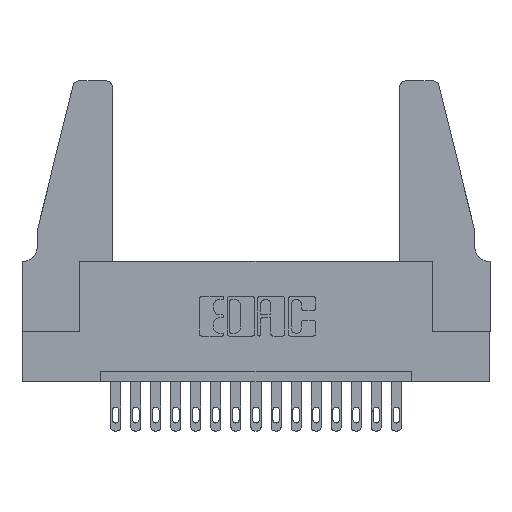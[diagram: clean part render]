
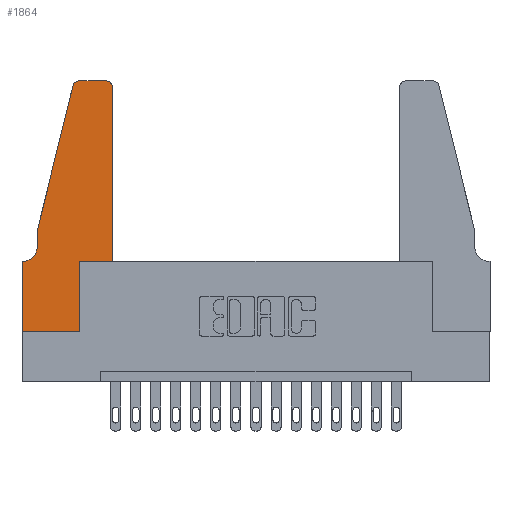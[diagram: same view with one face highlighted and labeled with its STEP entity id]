
A CAD part, top view. The second image highlights one B-rep face of the part: STEP entity #1864.
In plain terms, the highlighted planar face has unit normal (0, 0, 1).
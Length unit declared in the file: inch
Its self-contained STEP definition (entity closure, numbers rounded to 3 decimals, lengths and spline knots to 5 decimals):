
#254 = DIRECTION ( 'NONE',  ( 0., 1., 0. ) ) ;
#261 = VERTEX_POINT ( 'NONE', #9381 ) ;
#372 = VECTOR ( 'NONE', #9721, 39.37008 ) ;
#529 = EDGE_CURVE ( 'NONE', #10047, #14169, #13421, .T. ) ;
#622 = ORIENTED_EDGE ( 'NONE', *, *, #4790, .T. ) ;
#1301 = VERTEX_POINT ( 'NONE', #7020 ) ;
#1384 = CARTESIAN_POINT ( 'NONE',  ( 0.4505, 0.35, 0.37 ) ) ;
#1813 = LINE ( 'NONE', #4146, #16368 ) ;
#1864 = ADVANCED_FACE ( 'NONE', ( #2322 ), #10809, .T. ) ;
#1888 = DIRECTION ( 'NONE',  ( 0., -1., 0. ) ) ;
#2164 = DIRECTION ( 'NONE',  ( 0., 0., 1. ) ) ;
#2322 = FACE_OUTER_BOUND ( 'NONE', #7663, .T. ) ;
#2970 = DIRECTION ( 'NONE',  ( 1., 0., 0. ) ) ;
#3041 = VECTOR ( 'NONE', #2970, 39.37008 ) ;
#3191 = DIRECTION ( 'NONE',  ( 0., -1., 0. ) ) ;
#3827 = VERTEX_POINT ( 'NONE', #16383 ) ;
#4038 = CARTESIAN_POINT ( 'NONE',  ( 0.0755, 0.35, 0.37 ) ) ;
#4050 = VECTOR ( 'NONE', #8361, 39.37008 ) ;
#4146 = CARTESIAN_POINT ( 'NONE',  ( 0.2865, 0.35, 0.37 ) ) ;
#4230 = DIRECTION ( 'NONE',  ( 0., 0., 1. ) ) ;
#4712 = CIRCLE ( 'NONE', #5655, 0.07 ) ;
#4785 = EDGE_CURVE ( 'NONE', #4840, #15629, #5254, .T. ) ;
#4790 = EDGE_CURVE ( 'NONE', #15629, #10047, #1813, .T. ) ;
#4840 = VERTEX_POINT ( 'NONE', #9409 ) ;
#4907 = ORIENTED_EDGE ( 'NONE', *, *, #15145, .T. ) ;
#5006 = CARTESIAN_POINT ( 'NONE',  ( 0.4205, 1.22, 0.37 ) ) ;
#5213 = EDGE_CURVE ( 'NONE', #14169, #13486, #7251, .T. ) ;
#5254 = LINE ( 'NONE', #16036, #3041 ) ;
#5362 = DIRECTION ( 'NONE',  ( -1., 0., 0. ) ) ;
#5575 = ORIENTED_EDGE ( 'NONE', *, *, #11340, .T. ) ;
#5655 = AXIS2_PLACEMENT_3D ( 'NONE', #9706, #11009, #12337 ) ;
#5667 = CIRCLE ( 'NONE', #8144, 0.03 ) ;
#5766 = CARTESIAN_POINT ( 'NONE',  ( 0.25487, 1.22718, 0.37 ) ) ;
#6343 = ORIENTED_EDGE ( 'NONE', *, *, #11801, .T. ) ;
#6541 = EDGE_CURVE ( 'NONE', #15241, #4840, #14198, .T. ) ;
#6826 = ORIENTED_EDGE ( 'NONE', *, *, #14881, .T. ) ;
#7020 = CARTESIAN_POINT ( 'NONE',  ( 0.0055, 0.35, 0.37 ) ) ;
#7075 = CARTESIAN_POINT ( 'NONE',  ( 0.4205, 1.25, 0.37 ) ) ;
#7163 = CIRCLE ( 'NONE', #14122, 0.03 ) ;
#7246 = CARTESIAN_POINT ( 'NONE',  ( 0.2605, 1.25, 0.37 ) ) ;
#7251 = LINE ( 'NONE', #10369, #13852 ) ;
#7286 = CARTESIAN_POINT ( 'NONE',  ( 0.284, 1.22, 0.37 ) ) ;
#7649 = CARTESIAN_POINT ( 'NONE',  ( 0.4505, 1.22, 0.37 ) ) ;
#7663 = EDGE_LOOP ( 'NONE', ( #6343, #15482, #5575, #4907, #11288, #6826, #15366, #9174, #622, #8635, #10661, #15835 ) ) ;
#8144 = AXIS2_PLACEMENT_3D ( 'NONE', #5006, #11484, #16696 ) ;
#8361 = DIRECTION ( 'NONE',  ( -0.239, -0.971, 0. ) ) ;
#8538 = CARTESIAN_POINT ( 'NONE',  ( 0.0755, 0.5, 0.37 ) ) ;
#8635 = ORIENTED_EDGE ( 'NONE', *, *, #529, .T. ) ;
#8824 = LINE ( 'NONE', #8538, #16271 ) ;
#9174 = ORIENTED_EDGE ( 'NONE', *, *, #4785, .T. ) ;
#9213 = CARTESIAN_POINT ( 'NONE',  ( 0., 0.35, 0.37 ) ) ;
#9381 = CARTESIAN_POINT ( 'NONE',  ( 0.284, 1.25, 0.37 ) ) ;
#9409 = CARTESIAN_POINT ( 'NONE',  ( 0., 0., 0.37 ) ) ;
#9539 = CARTESIAN_POINT ( 'NONE',  ( 0.0755, 0.5, 0.37 ) ) ;
#9706 = CARTESIAN_POINT ( 'NONE',  ( 0.0055, 0.42, 0.37 ) ) ;
#9721 = DIRECTION ( 'NONE',  ( -1., 0., 0. ) ) ;
#9727 = CARTESIAN_POINT ( 'NONE',  ( 0.2865, 0., 0.37 ) ) ;
#10047 = VERTEX_POINT ( 'NONE', #16821 ) ;
#10242 = EDGE_CURVE ( 'NONE', #13486, #16090, #5667, .T. ) ;
#10304 = VECTOR ( 'NONE', #13217, 39.37008 ) ;
#10369 = CARTESIAN_POINT ( 'NONE',  ( 0.4505, 0.35, 0.37 ) ) ;
#10422 = DIRECTION ( 'NONE',  ( 0., 1., 0. ) ) ;
#10661 = ORIENTED_EDGE ( 'NONE', *, *, #5213, .T. ) ;
#10676 = VECTOR ( 'NONE', #3191, 39.37008 ) ;
#10809 = PLANE ( 'NONE',  #11166 ) ;
#10815 = LINE ( 'NONE', #9539, #4050 ) ;
#10983 = CARTESIAN_POINT ( 'NONE',  ( 0., 0.35, 0.37 ) ) ;
#11009 = DIRECTION ( 'NONE',  ( 0., 0., -1. ) ) ;
#11166 = AXIS2_PLACEMENT_3D ( 'NONE', #10983, #4230, #12257 ) ;
#11288 = ORIENTED_EDGE ( 'NONE', *, *, #15777, .T. ) ;
#11340 = EDGE_CURVE ( 'NONE', #13668, #3827, #10815, .T. ) ;
#11484 = DIRECTION ( 'NONE',  ( 0., 0., 1. ) ) ;
#11801 = EDGE_CURVE ( 'NONE', #16090, #261, #12048, .T. ) ;
#12048 = LINE ( 'NONE', #7246, #372 ) ;
#12094 = CARTESIAN_POINT ( 'NONE',  ( 0.0755, 0.42, 0.37 ) ) ;
#12257 = DIRECTION ( 'NONE',  ( 1., 0., 0. ) ) ;
#12337 = DIRECTION ( 'NONE',  ( -1., 0., 0. ) ) ;
#12630 = DIRECTION ( 'NONE',  ( 1., 0., 0. ) ) ;
#13188 = VECTOR ( 'NONE', #5362, 39.37008 ) ;
#13217 = DIRECTION ( 'NONE',  ( 1., 0., 0. ) ) ;
#13421 = LINE ( 'NONE', #1384, #10304 ) ;
#13486 = VERTEX_POINT ( 'NONE', #7649 ) ;
#13668 = VERTEX_POINT ( 'NONE', #5766 ) ;
#13852 = VECTOR ( 'NONE', #10422, 39.37008 ) ;
#14122 = AXIS2_PLACEMENT_3D ( 'NONE', #7286, #2164, #12630 ) ;
#14169 = VERTEX_POINT ( 'NONE', #16778 ) ;
#14198 = LINE ( 'NONE', #14761, #10676 ) ;
#14761 = CARTESIAN_POINT ( 'NONE',  ( 0., 0., 0.37 ) ) ;
#14881 = EDGE_CURVE ( 'NONE', #1301, #15241, #15018, .T. ) ;
#15018 = LINE ( 'NONE', #4038, #13188 ) ;
#15145 = EDGE_CURVE ( 'NONE', #3827, #15295, #8824, .T. ) ;
#15241 = VERTEX_POINT ( 'NONE', #9213 ) ;
#15295 = VERTEX_POINT ( 'NONE', #12094 ) ;
#15366 = ORIENTED_EDGE ( 'NONE', *, *, #6541, .T. ) ;
#15482 = ORIENTED_EDGE ( 'NONE', *, *, #15818, .T. ) ;
#15629 = VERTEX_POINT ( 'NONE', #9727 ) ;
#15777 = EDGE_CURVE ( 'NONE', #15295, #1301, #4712, .T. ) ;
#15818 = EDGE_CURVE ( 'NONE', #261, #13668, #7163, .T. ) ;
#15835 = ORIENTED_EDGE ( 'NONE', *, *, #10242, .T. ) ;
#16036 = CARTESIAN_POINT ( 'NONE',  ( 0., 0., 0.37 ) ) ;
#16090 = VERTEX_POINT ( 'NONE', #7075 ) ;
#16271 = VECTOR ( 'NONE', #1888, 39.37008 ) ;
#16368 = VECTOR ( 'NONE', #254, 39.37008 ) ;
#16383 = CARTESIAN_POINT ( 'NONE',  ( 0.0755, 0.5, 0.37 ) ) ;
#16696 = DIRECTION ( 'NONE',  ( 1., 0., 0. ) ) ;
#16778 = CARTESIAN_POINT ( 'NONE',  ( 0.4505, 0.35, 0.37 ) ) ;
#16821 = CARTESIAN_POINT ( 'NONE',  ( 0.2865, 0.35, 0.37 ) ) ;
